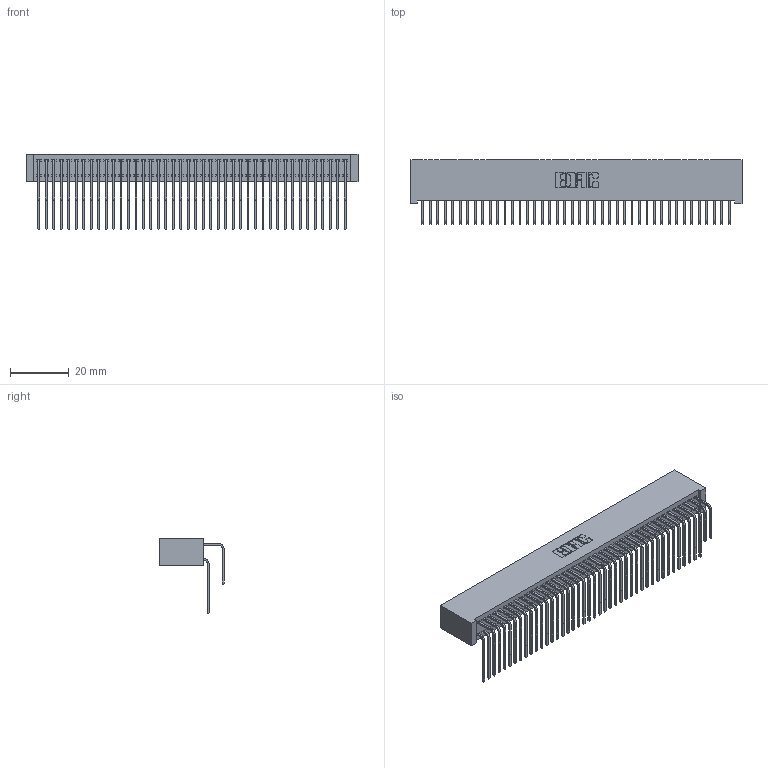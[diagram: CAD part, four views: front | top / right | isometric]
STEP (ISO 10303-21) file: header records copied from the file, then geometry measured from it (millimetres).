
FILE_DESCRIPTION (( 'STEP AP203' ), '1' );
FILE_NAME ('342-084-558-201.STEP', '2019-10-04T12:50:14', ( '' ), ( '' ), 'SwSTEP 2.0', 'SolidWorks 2016', '' );
FILE_SCHEMA (( 'CONFIG_CONTROL_DESIGN' ));
Length unit declared in the file: inch
Products named in the file (4): 342 Part_Lugless; 345-292-001_558 559 Tail - 1; 345-292-001_558 Tail - 2; 342-084-558-201
Assembly tree (85 placements, depth 2):
  342-084-558-201
    342 Part_Lugless
    345-292-001_558 559 Tail - 1  x42
    345-292-001_558 Tail - 2  x42
Bounding box: 112.93 x 21.91 x 25.78 mm (x, y, z)
Volume: 11070.7 mm3; surface area: 20658.6 mm2
Topology: 85 solids, 85 shells, 4638 faces, 13799 edges, 9086 vertices
Faces by surface type: plane 3254, cylinder 1384
Entity records: 28395 total; most frequent: CARTESIAN_POINT 4753, ORIENTED_EDGE 4638, DIRECTION 4035, EDGE_CURVE 2319, LINE 2159, VECTOR 2159, VERTEX_POINT 1542, AXIS2_PLACEMENT_3D 938
